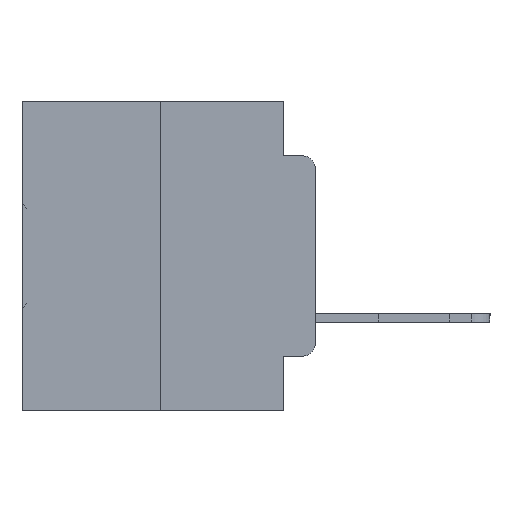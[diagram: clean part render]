
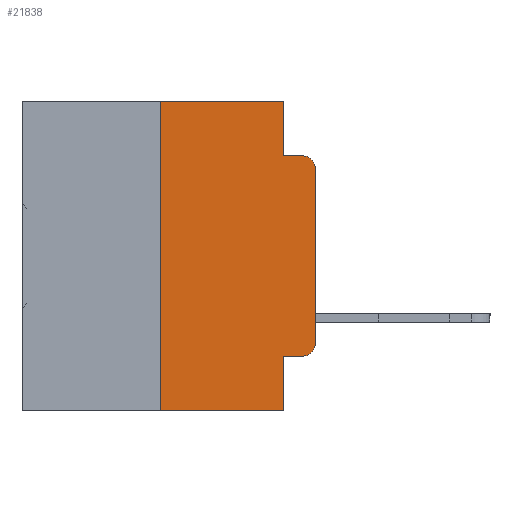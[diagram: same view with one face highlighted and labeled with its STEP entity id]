
A CAD part, left-side view. The second image highlights one B-rep face of the part: STEP entity #21838.
In plain terms, the highlighted planar face has unit normal (-1, 0, 0).
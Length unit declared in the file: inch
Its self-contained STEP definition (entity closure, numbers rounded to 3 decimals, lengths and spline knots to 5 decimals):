
#646 = VERTEX_POINT ( 'NONE', #8968 ) ;
#729 = DIRECTION ( 'NONE',  ( 0., 0., -1. ) ) ;
#1528 = CARTESIAN_POINT ( 'NONE',  ( 0., 0.051, -0.4115 ) ) ;
#1963 = VECTOR ( 'NONE', #15251, 39.37008 ) ;
#1968 = EDGE_CURVE ( 'NONE', #4860, #28406, #31962, .T. ) ;
#2486 = LINE ( 'NONE', #27579, #20824 ) ;
#2760 = LINE ( 'NONE', #26723, #21112 ) ;
#3195 = AXIS2_PLACEMENT_3D ( 'NONE', #24610, #9619, #27112 ) ;
#3453 = LINE ( 'NONE', #25876, #29257 ) ;
#3489 = DIRECTION ( 'NONE',  ( 0., -1., 0. ) ) ;
#3664 = CARTESIAN_POINT ( 'NONE',  ( 0., 0.02, -0.3915 ) ) ;
#4189 = CARTESIAN_POINT ( 'NONE',  ( 0., 0.25, 0. ) ) ;
#4860 = VERTEX_POINT ( 'NONE', #4189 ) ;
#4972 = EDGE_CURVE ( 'NONE', #21963, #24463, #21495, .T. ) ;
#4991 = CARTESIAN_POINT ( 'NONE',  ( 0., 0.25, -0.5 ) ) ;
#5983 = CARTESIAN_POINT ( 'NONE',  ( 0., 0., -0.1085 ) ) ;
#6151 = DIRECTION ( 'NONE',  ( 0., 0., -1. ) ) ;
#6497 = EDGE_CURVE ( 'NONE', #10427, #14820, #8611, .T. ) ;
#7162 = FACE_OUTER_BOUND ( 'NONE', #31893, .T. ) ;
#8611 = LINE ( 'NONE', #30264, #1963 ) ;
#8968 = CARTESIAN_POINT ( 'NONE',  ( 0., 0.02, -0.0885 ) ) ;
#9118 = VECTOR ( 'NONE', #22427, 39.37008 ) ;
#9298 = EDGE_CURVE ( 'NONE', #10427, #4860, #30001, .T. ) ;
#9619 = DIRECTION ( 'NONE',  ( -1., 0., 0. ) ) ;
#10427 = VERTEX_POINT ( 'NONE', #4991 ) ;
#10713 = PLANE ( 'NONE',  #28335 ) ;
#12077 = CARTESIAN_POINT ( 'NONE',  ( 0., 0.051, -0.0885 ) ) ;
#12479 = CARTESIAN_POINT ( 'NONE',  ( 0., 0.051, 0. ) ) ;
#12482 = CARTESIAN_POINT ( 'NONE',  ( 0., 0., -0.3915 ) ) ;
#12580 = DIRECTION ( 'NONE',  ( 0., 0., -1. ) ) ;
#13756 = CARTESIAN_POINT ( 'NONE',  ( 0., 0.02, -0.4115 ) ) ;
#14250 = DIRECTION ( 'NONE',  ( 0., 0., 1. ) ) ;
#14464 = VERTEX_POINT ( 'NONE', #1528 ) ;
#14654 = LINE ( 'NONE', #12077, #27974 ) ;
#14820 = VERTEX_POINT ( 'NONE', #30519 ) ;
#15251 = DIRECTION ( 'NONE',  ( 0., -1., 0. ) ) ;
#15708 = DIRECTION ( 'NONE',  ( 1., 0., 0. ) ) ;
#16530 = LINE ( 'NONE', #12479, #9118 ) ;
#18153 = CARTESIAN_POINT ( 'NONE',  ( 0., 0.051, -0.0885 ) ) ;
#18454 = ORIENTED_EDGE ( 'NONE', *, *, #9298, .F. ) ;
#20824 = VECTOR ( 'NONE', #12580, 39.37008 ) ;
#20912 = EDGE_CURVE ( 'NONE', #28891, #646, #14654, .T. ) ;
#21009 = AXIS2_PLACEMENT_3D ( 'NONE', #3664, #21104, #6151 ) ;
#21104 = DIRECTION ( 'NONE',  ( -1., 0., 0. ) ) ;
#21112 = VECTOR ( 'NONE', #14250, 39.37008 ) ;
#21127 = CARTESIAN_POINT ( 'NONE',  ( 0., 0.051, 0. ) ) ;
#21453 = ORIENTED_EDGE ( 'NONE', *, *, #24241, .T. ) ;
#21495 = CIRCLE ( 'NONE', #21009, 0.02 ) ;
#21526 = EDGE_CURVE ( 'NONE', #21906, #646, #24004, .T. ) ;
#21838 = ADVANCED_FACE ( 'NONE', ( #7162 ), #10713, .F. ) ;
#21906 = VERTEX_POINT ( 'NONE', #5983 ) ;
#21963 = VERTEX_POINT ( 'NONE', #13756 ) ;
#22427 = DIRECTION ( 'NONE',  ( 0., 0., -1. ) ) ;
#22648 = EDGE_CURVE ( 'NONE', #28406, #28891, #16530, .T. ) ;
#22679 = EDGE_CURVE ( 'NONE', #14464, #14820, #2486, .T. ) ;
#24004 = CIRCLE ( 'NONE', #3195, 0.02 ) ;
#24241 = EDGE_CURVE ( 'NONE', #24463, #21906, #2760, .T. ) ;
#24463 = VERTEX_POINT ( 'NONE', #12482 ) ;
#24610 = CARTESIAN_POINT ( 'NONE',  ( 0., 0.02, -0.1085 ) ) ;
#25262 = VECTOR ( 'NONE', #28076, 39.37008 ) ;
#25876 = CARTESIAN_POINT ( 'NONE',  ( 0., 0.051, -0.4115 ) ) ;
#26210 = ORIENTED_EDGE ( 'NONE', *, *, #20912, .F. ) ;
#26698 = ORIENTED_EDGE ( 'NONE', *, *, #6497, .T. ) ;
#26723 = CARTESIAN_POINT ( 'NONE',  ( 0., 0., 0. ) ) ;
#27112 = DIRECTION ( 'NONE',  ( 0., 0., -1. ) ) ;
#27449 = ORIENTED_EDGE ( 'NONE', *, *, #22648, .F. ) ;
#27579 = CARTESIAN_POINT ( 'NONE',  ( 0., 0.051, 0. ) ) ;
#27974 = VECTOR ( 'NONE', #29576, 39.37008 ) ;
#28020 = CARTESIAN_POINT ( 'NONE',  ( 0., 0.25, 0. ) ) ;
#28076 = DIRECTION ( 'NONE',  ( 0., -1., 0. ) ) ;
#28330 = ORIENTED_EDGE ( 'NONE', *, *, #31777, .T. ) ;
#28335 = AXIS2_PLACEMENT_3D ( 'NONE', #30746, #15708, #729 ) ;
#28406 = VERTEX_POINT ( 'NONE', #21127 ) ;
#28721 = ORIENTED_EDGE ( 'NONE', *, *, #4972, .T. ) ;
#28891 = VERTEX_POINT ( 'NONE', #18153 ) ;
#29206 = VECTOR ( 'NONE', #30565, 39.37008 ) ;
#29257 = VECTOR ( 'NONE', #3489, 39.37008 ) ;
#29444 = ORIENTED_EDGE ( 'NONE', *, *, #1968, .F. ) ;
#29576 = DIRECTION ( 'NONE',  ( 0., -1., 0. ) ) ;
#30001 = LINE ( 'NONE', #28020, #29206 ) ;
#30135 = ORIENTED_EDGE ( 'NONE', *, *, #21526, .T. ) ;
#30162 = CARTESIAN_POINT ( 'NONE',  ( 0., 0.473, 0. ) ) ;
#30264 = CARTESIAN_POINT ( 'NONE',  ( 0., 0.473, -0.5 ) ) ;
#30519 = CARTESIAN_POINT ( 'NONE',  ( 0., 0.051, -0.5 ) ) ;
#30565 = DIRECTION ( 'NONE',  ( 0., 0., 1. ) ) ;
#30746 = CARTESIAN_POINT ( 'NONE',  ( 0., 0.473, 0. ) ) ;
#31398 = ORIENTED_EDGE ( 'NONE', *, *, #22679, .F. ) ;
#31777 = EDGE_CURVE ( 'NONE', #14464, #21963, #3453, .T. ) ;
#31893 = EDGE_LOOP ( 'NONE', ( #21453, #30135, #26210, #27449, #29444, #18454, #26698, #31398, #28330, #28721 ) ) ;
#31962 = LINE ( 'NONE', #30162, #25262 ) ;
